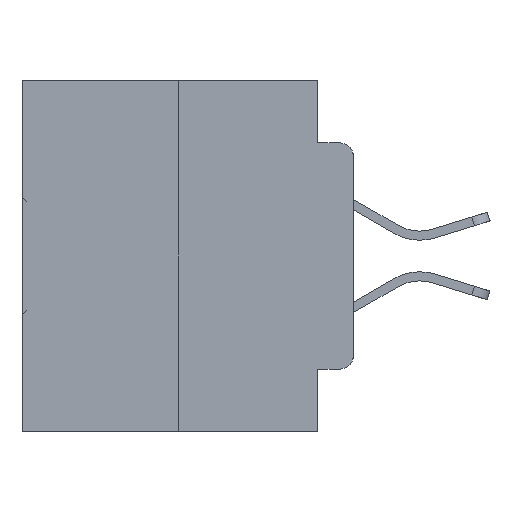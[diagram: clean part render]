
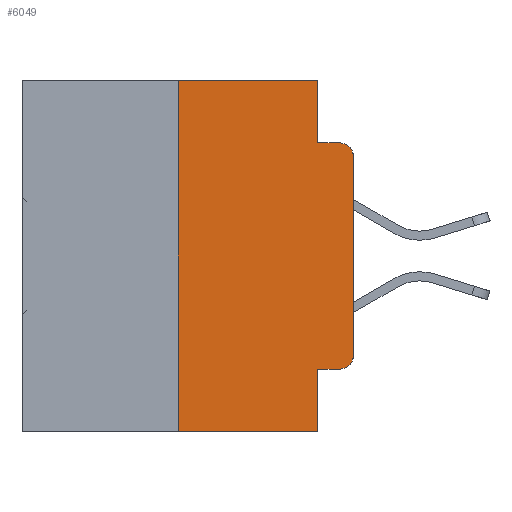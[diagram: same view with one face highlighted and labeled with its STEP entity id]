
A CAD part, left-side view. The second image highlights one B-rep face of the part: STEP entity #6049.
In plain terms, the highlighted planar face has unit normal (-1, 0, 0).
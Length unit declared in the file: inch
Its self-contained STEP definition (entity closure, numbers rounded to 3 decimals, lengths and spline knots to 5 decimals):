
#831 = VERTEX_POINT ( 'NONE', #18845 ) ;
#1553 = VECTOR ( 'NONE', #14168, 39.37008 ) ;
#2213 = VECTOR ( 'NONE', #17516, 39.37008 ) ;
#2657 = EDGE_CURVE ( 'NONE', #14241, #21538, #4166, .T. ) ;
#2686 = ORIENTED_EDGE ( 'NONE', *, *, #2657, .F. ) ;
#3075 = VERTEX_POINT ( 'NONE', #9525 ) ;
#3300 = ORIENTED_EDGE ( 'NONE', *, *, #28399, .T. ) ;
#3312 = CARTESIAN_POINT ( 'NONE',  ( 0., 0., 0. ) ) ;
#3578 = CARTESIAN_POINT ( 'NONE',  ( 0., 0., -0.1085 ) ) ;
#3976 = EDGE_CURVE ( 'NONE', #831, #8395, #13445, .T. ) ;
#4070 = EDGE_CURVE ( 'NONE', #20303, #3075, #7129, .T. ) ;
#4166 = LINE ( 'NONE', #27797, #2213 ) ;
#4217 = DIRECTION ( 'NONE',  ( 0., -1., 0. ) ) ;
#4546 = PLANE ( 'NONE',  #25661 ) ;
#5205 = ORIENTED_EDGE ( 'NONE', *, *, #14518, .T. ) ;
#5868 = LINE ( 'NONE', #24447, #28873 ) ;
#5893 = AXIS2_PLACEMENT_3D ( 'NONE', #23763, #13775, #16334 ) ;
#6003 = CARTESIAN_POINT ( 'NONE',  ( 0., 0.02, -0.3915 ) ) ;
#6013 = ORIENTED_EDGE ( 'NONE', *, *, #4070, .F. ) ;
#6049 = ADVANCED_FACE ( 'NONE', ( #32358 ), #4546, .F. ) ;
#6544 = CARTESIAN_POINT ( 'NONE',  ( 0., 0.051, -0.4115 ) ) ;
#7087 = CARTESIAN_POINT ( 'NONE',  ( 0., 0.473, 0. ) ) ;
#7129 = LINE ( 'NONE', #9740, #1553 ) ;
#7171 = AXIS2_PLACEMENT_3D ( 'NONE', #6003, #8871, #13541 ) ;
#7643 = DIRECTION ( 'NONE',  ( 0., 0., 1. ) ) ;
#8395 = VERTEX_POINT ( 'NONE', #23181 ) ;
#8726 = LINE ( 'NONE', #10906, #30959 ) ;
#8871 = DIRECTION ( 'NONE',  ( -1., 0., 0. ) ) ;
#9153 = CARTESIAN_POINT ( 'NONE',  ( 0., 0.051, 0. ) ) ;
#9525 = CARTESIAN_POINT ( 'NONE',  ( 0., 0.051, 0. ) ) ;
#9661 = DIRECTION ( 'NONE',  ( 1., 0., 0. ) ) ;
#9739 = CARTESIAN_POINT ( 'NONE',  ( 0., 0.02, -0.4115 ) ) ;
#9740 = CARTESIAN_POINT ( 'NONE',  ( 0., 0.473, 0. ) ) ;
#9987 = ORIENTED_EDGE ( 'NONE', *, *, #12377, .T. ) ;
#10099 = EDGE_CURVE ( 'NONE', #30645, #31345, #5868, .T. ) ;
#10906 = CARTESIAN_POINT ( 'NONE',  ( 0., 0.25, 0. ) ) ;
#11584 = ORIENTED_EDGE ( 'NONE', *, *, #3976, .T. ) ;
#12153 = ORIENTED_EDGE ( 'NONE', *, *, #14438, .F. ) ;
#12202 = DIRECTION ( 'NONE',  ( 0., 0., -1. ) ) ;
#12377 = EDGE_CURVE ( 'NONE', #20269, #29993, #25547, .T. ) ;
#12389 = ORIENTED_EDGE ( 'NONE', *, *, #10099, .T. ) ;
#12413 = LINE ( 'NONE', #9153, #29463 ) ;
#13445 = LINE ( 'NONE', #31159, #22216 ) ;
#13541 = DIRECTION ( 'NONE',  ( 0., 0., -1. ) ) ;
#13775 = DIRECTION ( 'NONE',  ( -1., 0., 0. ) ) ;
#14160 = EDGE_LOOP ( 'NONE', ( #9987, #5205, #2686, #23203, #6013, #12153, #11584, #27119, #12389, #3300 ) ) ;
#14168 = DIRECTION ( 'NONE',  ( 0., -1., 0. ) ) ;
#14241 = VERTEX_POINT ( 'NONE', #30450 ) ;
#14438 = EDGE_CURVE ( 'NONE', #831, #20303, #8726, .T. ) ;
#14518 = EDGE_CURVE ( 'NONE', #29993, #21538, #14660, .T. ) ;
#14660 = CIRCLE ( 'NONE', #5893, 0.02 ) ;
#15136 = VECTOR ( 'NONE', #32660, 39.37008 ) ;
#16334 = DIRECTION ( 'NONE',  ( 0., 0., -1. ) ) ;
#17516 = DIRECTION ( 'NONE',  ( 0., -1., 0. ) ) ;
#17606 = CARTESIAN_POINT ( 'NONE',  ( 0., 0., -0.3915 ) ) ;
#18845 = CARTESIAN_POINT ( 'NONE',  ( 0., 0.25, -0.5 ) ) ;
#20269 = VERTEX_POINT ( 'NONE', #17606 ) ;
#20303 = VERTEX_POINT ( 'NONE', #27890 ) ;
#21538 = VERTEX_POINT ( 'NONE', #27920 ) ;
#22216 = VECTOR ( 'NONE', #28471, 39.37008 ) ;
#23181 = CARTESIAN_POINT ( 'NONE',  ( 0., 0.051, -0.5 ) ) ;
#23203 = ORIENTED_EDGE ( 'NONE', *, *, #29600, .F. ) ;
#23449 = LINE ( 'NONE', #24833, #15136 ) ;
#23763 = CARTESIAN_POINT ( 'NONE',  ( 0., 0.02, -0.1085 ) ) ;
#24241 = EDGE_CURVE ( 'NONE', #30645, #8395, #12413, .T. ) ;
#24447 = CARTESIAN_POINT ( 'NONE',  ( 0., 0.051, -0.4115 ) ) ;
#24492 = DIRECTION ( 'NONE',  ( 0., 0., -1. ) ) ;
#24833 = CARTESIAN_POINT ( 'NONE',  ( 0., 0.051, 0. ) ) ;
#25547 = LINE ( 'NONE', #3312, #29537 ) ;
#25661 = AXIS2_PLACEMENT_3D ( 'NONE', #7087, #9661, #12202 ) ;
#26199 = DIRECTION ( 'NONE',  ( 0., 0., 1. ) ) ;
#27119 = ORIENTED_EDGE ( 'NONE', *, *, #24241, .F. ) ;
#27797 = CARTESIAN_POINT ( 'NONE',  ( 0., 0.051, -0.0885 ) ) ;
#27890 = CARTESIAN_POINT ( 'NONE',  ( 0., 0.25, 0. ) ) ;
#27920 = CARTESIAN_POINT ( 'NONE',  ( 0., 0.02, -0.0885 ) ) ;
#28399 = EDGE_CURVE ( 'NONE', #31345, #20269, #28760, .T. ) ;
#28471 = DIRECTION ( 'NONE',  ( 0., -1., 0. ) ) ;
#28760 = CIRCLE ( 'NONE', #7171, 0.02 ) ;
#28873 = VECTOR ( 'NONE', #4217, 39.37008 ) ;
#29463 = VECTOR ( 'NONE', #24492, 39.37008 ) ;
#29537 = VECTOR ( 'NONE', #7643, 39.37008 ) ;
#29600 = EDGE_CURVE ( 'NONE', #3075, #14241, #23449, .T. ) ;
#29993 = VERTEX_POINT ( 'NONE', #3578 ) ;
#30450 = CARTESIAN_POINT ( 'NONE',  ( 0., 0.051, -0.0885 ) ) ;
#30645 = VERTEX_POINT ( 'NONE', #6544 ) ;
#30959 = VECTOR ( 'NONE', #26199, 39.37008 ) ;
#31159 = CARTESIAN_POINT ( 'NONE',  ( 0., 0.473, -0.5 ) ) ;
#31345 = VERTEX_POINT ( 'NONE', #9739 ) ;
#32358 = FACE_OUTER_BOUND ( 'NONE', #14160, .T. ) ;
#32660 = DIRECTION ( 'NONE',  ( 0., 0., -1. ) ) ;
